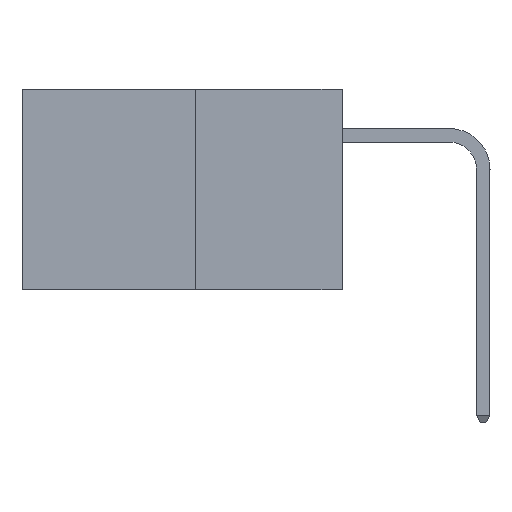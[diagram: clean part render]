
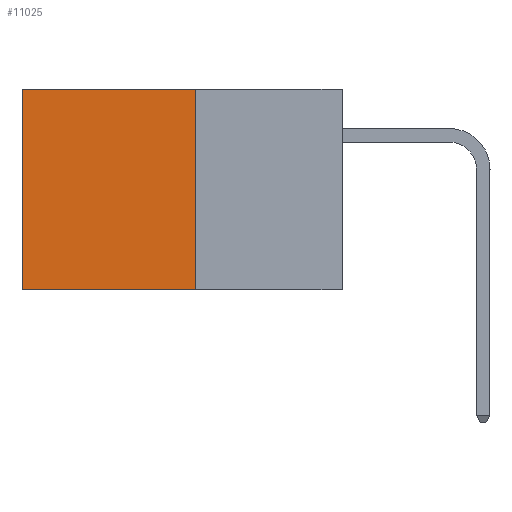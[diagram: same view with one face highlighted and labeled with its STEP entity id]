
A CAD part, left-side view. The second image highlights one B-rep face of the part: STEP entity #11025.
In plain terms, the highlighted planar face has unit normal (-1, 0, 0).
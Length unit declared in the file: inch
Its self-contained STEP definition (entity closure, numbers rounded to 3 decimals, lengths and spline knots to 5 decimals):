
#1739 = CARTESIAN_POINT ( 'NONE',  ( 0.277, 0.59, -0.37 ) ) ;
#2398 = CARTESIAN_POINT ( 'NONE',  ( 0.277, 0.59, -0.37 ) ) ;
#2476 = ORIENTED_EDGE ( 'NONE', *, *, #3619, .T. ) ;
#3553 = DIRECTION ( 'NONE',  ( 1., 0., 0. ) ) ;
#3619 = EDGE_CURVE ( 'NONE', #31500, #13129, #25895, .T. ) ;
#6787 = AXIS2_PLACEMENT_3D ( 'NONE', #28698, #3553, #21221 ) ;
#6800 = CARTESIAN_POINT ( 'NONE',  ( 0.277, 0.27, 0. ) ) ;
#8686 = CARTESIAN_POINT ( 'NONE',  ( 0.277, 0.27, -0.37 ) ) ;
#10036 = DIRECTION ( 'NONE',  ( 0., 0., -1. ) ) ;
#11025 = ADVANCED_FACE ( 'NONE', ( #20211 ), #18667, .F. ) ;
#11228 = DIRECTION ( 'NONE',  ( 0., 1., 0. ) ) ;
#12149 = CARTESIAN_POINT ( 'NONE',  ( 0.277, 0.59, 0. ) ) ;
#12484 = VECTOR ( 'NONE', #31975, 39.37008 ) ;
#13129 = VERTEX_POINT ( 'NONE', #12149 ) ;
#13998 = VECTOR ( 'NONE', #10036, 39.37008 ) ;
#14669 = ORIENTED_EDGE ( 'NONE', *, *, #31363, .F. ) ;
#15575 = LINE ( 'NONE', #2398, #13998 ) ;
#16079 = CARTESIAN_POINT ( 'NONE',  ( 0.277, 0.27, 0. ) ) ;
#16381 = CARTESIAN_POINT ( 'NONE',  ( 0.277, 0.27, -0.37 ) ) ;
#18044 = DIRECTION ( 'NONE',  ( 0., 0., -1. ) ) ;
#18667 = PLANE ( 'NONE',  #6787 ) ;
#19495 = VERTEX_POINT ( 'NONE', #1739 ) ;
#20211 = FACE_OUTER_BOUND ( 'NONE', #22722, .T. ) ;
#20920 = VECTOR ( 'NONE', #11228, 39.37008 ) ;
#21221 = DIRECTION ( 'NONE',  ( 0., 0., -1. ) ) ;
#21546 = LINE ( 'NONE', #30573, #29018 ) ;
#22722 = EDGE_LOOP ( 'NONE', ( #28772, #27879, #14669, #2476 ) ) ;
#24232 = VERTEX_POINT ( 'NONE', #16381 ) ;
#25895 = LINE ( 'NONE', #6800, #12484 ) ;
#27618 = LINE ( 'NONE', #8686, #20920 ) ;
#27879 = ORIENTED_EDGE ( 'NONE', *, *, #30264, .F. ) ;
#27979 = EDGE_CURVE ( 'NONE', #13129, #19495, #15575, .T. ) ;
#28698 = CARTESIAN_POINT ( 'NONE',  ( 0.277, 0.27, -0.37 ) ) ;
#28772 = ORIENTED_EDGE ( 'NONE', *, *, #27979, .T. ) ;
#29018 = VECTOR ( 'NONE', #18044, 39.37008 ) ;
#30264 = EDGE_CURVE ( 'NONE', #24232, #19495, #27618, .T. ) ;
#30573 = CARTESIAN_POINT ( 'NONE',  ( 0.277, 0.27, -0.37 ) ) ;
#31363 = EDGE_CURVE ( 'NONE', #31500, #24232, #21546, .T. ) ;
#31500 = VERTEX_POINT ( 'NONE', #16079 ) ;
#31975 = DIRECTION ( 'NONE',  ( 0., 1., 0. ) ) ;
